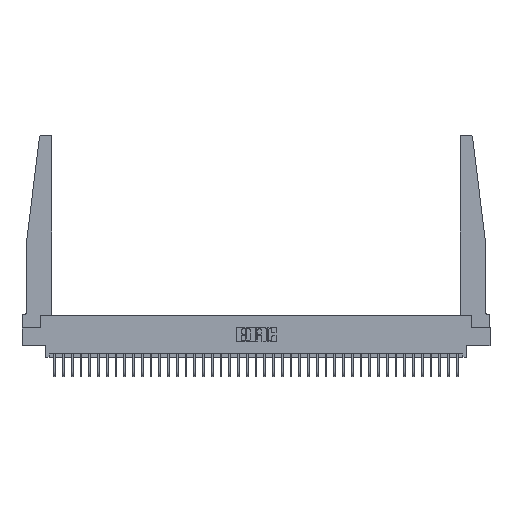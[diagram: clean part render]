
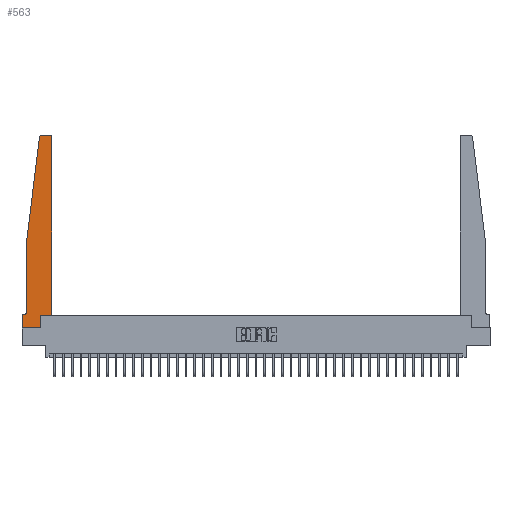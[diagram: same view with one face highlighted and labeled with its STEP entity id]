
A CAD part, top view. The second image highlights one B-rep face of the part: STEP entity #563.
In plain terms, the highlighted planar face has unit normal (0, 0, 1).
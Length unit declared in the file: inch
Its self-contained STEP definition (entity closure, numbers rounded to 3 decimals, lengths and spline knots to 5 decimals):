
#536 = VERTEX_POINT ( 'NONE', #32059 ) ;
#563 = ADVANCED_FACE ( 'NONE', ( #31840 ), #24367, .T. ) ;
#761 = EDGE_CURVE ( 'NONE', #26810, #27064, #4775, .T. ) ;
#1159 = VECTOR ( 'NONE', #1563, 39.37008 ) ;
#1244 = DIRECTION ( 'NONE',  ( 1., 0., 0. ) ) ;
#1563 = DIRECTION ( 'NONE',  ( -0.122, -0.992, 0. ) ) ;
#1694 = VERTEX_POINT ( 'NONE', #23507 ) ;
#2175 = EDGE_LOOP ( 'NONE', ( #16737, #2571, #5083, #12391, #17674, #25879, #27508, #8626, #19695, #10087, #28621, #13924 ) ) ;
#2247 = VERTEX_POINT ( 'NONE', #28219 ) ;
#2359 = EDGE_CURVE ( 'NONE', #27064, #2247, #9086, .T. ) ;
#2571 = ORIENTED_EDGE ( 'NONE', *, *, #15392, .T. ) ;
#2771 = VERTEX_POINT ( 'NONE', #24858 ) ;
#2848 = CARTESIAN_POINT ( 'NONE',  ( 0.25, 2.75, 0.37 ) ) ;
#3251 = EDGE_CURVE ( 'NONE', #5134, #11094, #10619, .T. ) ;
#3274 = LINE ( 'NONE', #21844, #29931 ) ;
#3346 = VERTEX_POINT ( 'NONE', #4184 ) ;
#4184 = CARTESIAN_POINT ( 'NONE',  ( 0.065, 0.2375, 0.37 ) ) ;
#4320 = LINE ( 'NONE', #27087, #30975 ) ;
#4593 = CIRCLE ( 'NONE', #12976, 0.03 ) ;
#4775 = CIRCLE ( 'NONE', #10759, 0.03 ) ;
#5064 = CARTESIAN_POINT ( 'NONE',  ( 0.24675, 2.72367, 0.37 ) ) ;
#5083 = ORIENTED_EDGE ( 'NONE', *, *, #18212, .T. ) ;
#5134 = VERTEX_POINT ( 'NONE', #14588 ) ;
#6017 = CARTESIAN_POINT ( 'NONE',  ( 0.395, 2.75, 0.37 ) ) ;
#8050 = LINE ( 'NONE', #19624, #1159 ) ;
#8626 = ORIENTED_EDGE ( 'NONE', *, *, #24939, .T. ) ;
#8953 = CARTESIAN_POINT ( 'NONE',  ( 0., 0.1875, 0.37 ) ) ;
#9086 = LINE ( 'NONE', #2848, #9901 ) ;
#9841 = CARTESIAN_POINT ( 'NONE',  ( 0.395, 2.72, 0.37 ) ) ;
#9901 = VECTOR ( 'NONE', #13122, 39.37008 ) ;
#10076 = CARTESIAN_POINT ( 'NONE',  ( 0.27653, 2.72, 0.37 ) ) ;
#10087 = ORIENTED_EDGE ( 'NONE', *, *, #11450, .T. ) ;
#10619 = LINE ( 'NONE', #14253, #25127 ) ;
#10751 = VERTEX_POINT ( 'NONE', #16499 ) ;
#10759 = AXIS2_PLACEMENT_3D ( 'NONE', #9841, #27857, #12434 ) ;
#11094 = VERTEX_POINT ( 'NONE', #19999 ) ;
#11450 = EDGE_CURVE ( 'NONE', #1694, #19187, #4320, .T. ) ;
#12051 = DIRECTION ( 'NONE',  ( 0., 0., -1. ) ) ;
#12171 = EDGE_CURVE ( 'NONE', #10751, #1694, #32126, .T. ) ;
#12391 = ORIENTED_EDGE ( 'NONE', *, *, #32435, .T. ) ;
#12394 = CARTESIAN_POINT ( 'NONE',  ( 0.425, 2.72, 0.37 ) ) ;
#12434 = DIRECTION ( 'NONE',  ( 1., 0., 0. ) ) ;
#12658 = DIRECTION ( 'NONE',  ( 1., 0., 0. ) ) ;
#12976 = AXIS2_PLACEMENT_3D ( 'NONE', #10076, #28087, #12658 ) ;
#13122 = DIRECTION ( 'NONE',  ( -1., 0., 0. ) ) ;
#13924 = ORIENTED_EDGE ( 'NONE', *, *, #761, .T. ) ;
#14253 = CARTESIAN_POINT ( 'NONE',  ( 0., 0., 0.37 ) ) ;
#14588 = CARTESIAN_POINT ( 'NONE',  ( 0., 0.1875, 0.37 ) ) ;
#15392 = EDGE_CURVE ( 'NONE', #2247, #28241, #4593, .T. ) ;
#16499 = CARTESIAN_POINT ( 'NONE',  ( 0.2605, 0., 0.37 ) ) ;
#16585 = DIRECTION ( 'NONE',  ( 0., -1., 0. ) ) ;
#16665 = VECTOR ( 'NONE', #16585, 39.37008 ) ;
#16727 = DIRECTION ( 'NONE',  ( 0., 0., 1. ) ) ;
#16737 = ORIENTED_EDGE ( 'NONE', *, *, #2359, .T. ) ;
#16802 = DIRECTION ( 'NONE',  ( -1., 0., 0. ) ) ;
#17008 = EDGE_CURVE ( 'NONE', #536, #5134, #3274, .T. ) ;
#17674 = ORIENTED_EDGE ( 'NONE', *, *, #23836, .T. ) ;
#17815 = AXIS2_PLACEMENT_3D ( 'NONE', #27481, #12051, #30101 ) ;
#18001 = DIRECTION ( 'NONE',  ( 0., 1., 0. ) ) ;
#18212 = EDGE_CURVE ( 'NONE', #28241, #2771, #8050, .T. ) ;
#18248 = LINE ( 'NONE', #29436, #16665 ) ;
#19015 = EDGE_CURVE ( 'NONE', #19187, #26810, #31801, .T. ) ;
#19187 = VERTEX_POINT ( 'NONE', #31526 ) ;
#19624 = CARTESIAN_POINT ( 'NONE',  ( 0.065, 1.25, 0.37 ) ) ;
#19634 = DIRECTION ( 'NONE',  ( 1., 0., 0. ) ) ;
#19695 = ORIENTED_EDGE ( 'NONE', *, *, #12171, .T. ) ;
#19999 = CARTESIAN_POINT ( 'NONE',  ( 0., 0., 0.37 ) ) ;
#21844 = CARTESIAN_POINT ( 'NONE',  ( 0.065, 0.1875, 0.37 ) ) ;
#22089 = DIRECTION ( 'NONE',  ( 0., 1., 0. ) ) ;
#22436 = CIRCLE ( 'NONE', #17815, 0.05 ) ;
#22831 = VECTOR ( 'NONE', #22089, 39.37008 ) ;
#23507 = CARTESIAN_POINT ( 'NONE',  ( 0.2605, 0.18, 0.37 ) ) ;
#23836 = EDGE_CURVE ( 'NONE', #3346, #536, #22436, .T. ) ;
#24365 = LINE ( 'NONE', #29913, #28816 ) ;
#24367 = PLANE ( 'NONE',  #25209 ) ;
#24858 = CARTESIAN_POINT ( 'NONE',  ( 0.065, 1.25, 0.37 ) ) ;
#24939 = EDGE_CURVE ( 'NONE', #11094, #10751, #24365, .T. ) ;
#25127 = VECTOR ( 'NONE', #32280, 39.37008 ) ;
#25209 = AXIS2_PLACEMENT_3D ( 'NONE', #8953, #16727, #1244 ) ;
#25879 = ORIENTED_EDGE ( 'NONE', *, *, #17008, .T. ) ;
#26810 = VERTEX_POINT ( 'NONE', #12394 ) ;
#27064 = VERTEX_POINT ( 'NONE', #6017 ) ;
#27087 = CARTESIAN_POINT ( 'NONE',  ( 0.425, 0.18, 0.37 ) ) ;
#27481 = CARTESIAN_POINT ( 'NONE',  ( 0.015, 0.2375, 0.37 ) ) ;
#27508 = ORIENTED_EDGE ( 'NONE', *, *, #3251, .T. ) ;
#27857 = DIRECTION ( 'NONE',  ( 0., 0., 1. ) ) ;
#28087 = DIRECTION ( 'NONE',  ( 0., 0., 1. ) ) ;
#28219 = CARTESIAN_POINT ( 'NONE',  ( 0.27653, 2.75, 0.37 ) ) ;
#28241 = VERTEX_POINT ( 'NONE', #5064 ) ;
#28621 = ORIENTED_EDGE ( 'NONE', *, *, #19015, .T. ) ;
#28816 = VECTOR ( 'NONE', #19634, 39.37008 ) ;
#29436 = CARTESIAN_POINT ( 'NONE',  ( 0.065, 1.25, 0.37 ) ) ;
#29706 = DIRECTION ( 'NONE',  ( 1., 0., 0. ) ) ;
#29777 = CARTESIAN_POINT ( 'NONE',  ( 0.2605, 0.18, 0.37 ) ) ;
#29913 = CARTESIAN_POINT ( 'NONE',  ( 0., 0., 0.37 ) ) ;
#29931 = VECTOR ( 'NONE', #16802, 39.37008 ) ;
#30101 = DIRECTION ( 'NONE',  ( -1., 0., 0. ) ) ;
#30193 = VECTOR ( 'NONE', #18001, 39.37008 ) ;
#30886 = CARTESIAN_POINT ( 'NONE',  ( 0.425, 0.18, 0.37 ) ) ;
#30975 = VECTOR ( 'NONE', #29706, 39.37008 ) ;
#31526 = CARTESIAN_POINT ( 'NONE',  ( 0.425, 0.18, 0.37 ) ) ;
#31801 = LINE ( 'NONE', #30886, #30193 ) ;
#31840 = FACE_OUTER_BOUND ( 'NONE', #2175, .T. ) ;
#32059 = CARTESIAN_POINT ( 'NONE',  ( 0.015, 0.1875, 0.37 ) ) ;
#32126 = LINE ( 'NONE', #29777, #22831 ) ;
#32280 = DIRECTION ( 'NONE',  ( 0., -1., 0. ) ) ;
#32435 = EDGE_CURVE ( 'NONE', #2771, #3346, #18248, .T. ) ;
